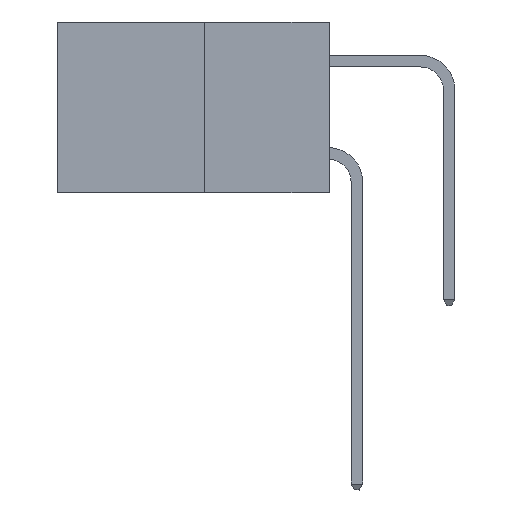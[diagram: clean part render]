
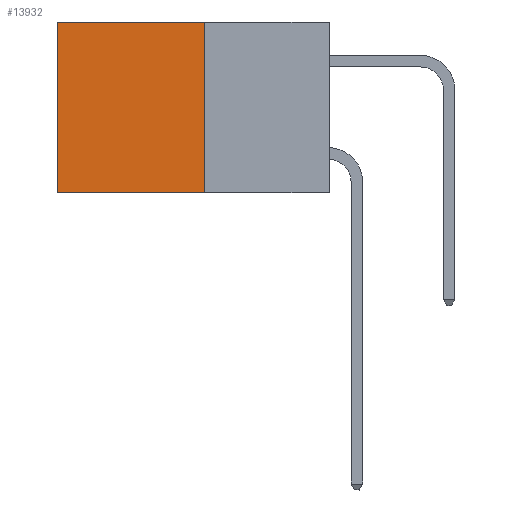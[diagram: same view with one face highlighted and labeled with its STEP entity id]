
A CAD part, left-side view. The second image highlights one B-rep face of the part: STEP entity #13932.
In plain terms, the highlighted planar face has unit normal (-1, 0, 0).
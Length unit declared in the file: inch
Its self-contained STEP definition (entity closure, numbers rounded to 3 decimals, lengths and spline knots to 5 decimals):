
#859 = LINE ( 'NONE', #13200, #6631 ) ;
#1654 = VERTEX_POINT ( 'NONE', #7100 ) ;
#1967 = FACE_OUTER_BOUND ( 'NONE', #4997, .T. ) ;
#3292 = CARTESIAN_POINT ( 'NONE',  ( 0.277, 0.59, -0.37 ) ) ;
#3707 = VECTOR ( 'NONE', #12489, 39.37008 ) ;
#3709 = ORIENTED_EDGE ( 'NONE', *, *, #13930, .T. ) ;
#3983 = ORIENTED_EDGE ( 'NONE', *, *, #11070, .F. ) ;
#4122 = ORIENTED_EDGE ( 'NONE', *, *, #5745, .F. ) ;
#4308 = ORIENTED_EDGE ( 'NONE', *, *, #6940, .T. ) ;
#4554 = VERTEX_POINT ( 'NONE', #12907 ) ;
#4997 = EDGE_LOOP ( 'NONE', ( #3709, #3983, #4122, #4308 ) ) ;
#5325 = CARTESIAN_POINT ( 'NONE',  ( 0.277, 0.27, 0. ) ) ;
#5418 = DIRECTION ( 'NONE',  ( 0., 0., -1. ) ) ;
#5628 = DIRECTION ( 'NONE',  ( 1., 0., 0. ) ) ;
#5721 = CARTESIAN_POINT ( 'NONE',  ( 0.277, 0.27, -0.37 ) ) ;
#5745 = EDGE_CURVE ( 'NONE', #5775, #1654, #5759, .T. ) ;
#5759 = LINE ( 'NONE', #5721, #14025 ) ;
#5775 = VERTEX_POINT ( 'NONE', #5325 ) ;
#6050 = LINE ( 'NONE', #11446, #3707 ) ;
#6631 = VECTOR ( 'NONE', #14227, 39.37008 ) ;
#6940 = EDGE_CURVE ( 'NONE', #5775, #4554, #859, .T. ) ;
#7100 = CARTESIAN_POINT ( 'NONE',  ( 0.277, 0.27, -0.37 ) ) ;
#8897 = PLANE ( 'NONE',  #9119 ) ;
#9119 = AXIS2_PLACEMENT_3D ( 'NONE', #12135, #5628, #13183 ) ;
#10350 = VERTEX_POINT ( 'NONE', #13497 ) ;
#10954 = LINE ( 'NONE', #3292, #13723 ) ;
#11070 = EDGE_CURVE ( 'NONE', #1654, #10350, #6050, .T. ) ;
#11087 = DIRECTION ( 'NONE',  ( 0., 0., -1. ) ) ;
#11446 = CARTESIAN_POINT ( 'NONE',  ( 0.277, 0.27, -0.37 ) ) ;
#12135 = CARTESIAN_POINT ( 'NONE',  ( 0.277, 0.27, -0.37 ) ) ;
#12489 = DIRECTION ( 'NONE',  ( 0., 1., 0. ) ) ;
#12907 = CARTESIAN_POINT ( 'NONE',  ( 0.277, 0.59, 0. ) ) ;
#13183 = DIRECTION ( 'NONE',  ( 0., 0., -1. ) ) ;
#13200 = CARTESIAN_POINT ( 'NONE',  ( 0.277, 0.27, 0. ) ) ;
#13497 = CARTESIAN_POINT ( 'NONE',  ( 0.277, 0.59, -0.37 ) ) ;
#13723 = VECTOR ( 'NONE', #11087, 39.37008 ) ;
#13930 = EDGE_CURVE ( 'NONE', #4554, #10350, #10954, .T. ) ;
#13932 = ADVANCED_FACE ( 'NONE', ( #1967 ), #8897, .F. ) ;
#14025 = VECTOR ( 'NONE', #5418, 39.37008 ) ;
#14227 = DIRECTION ( 'NONE',  ( 0., 1., 0. ) ) ;
